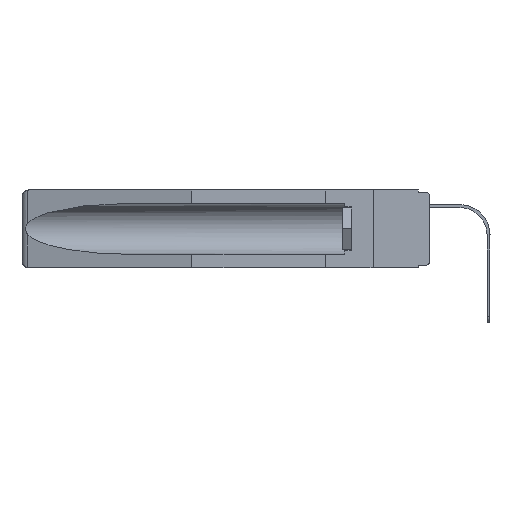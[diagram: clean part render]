
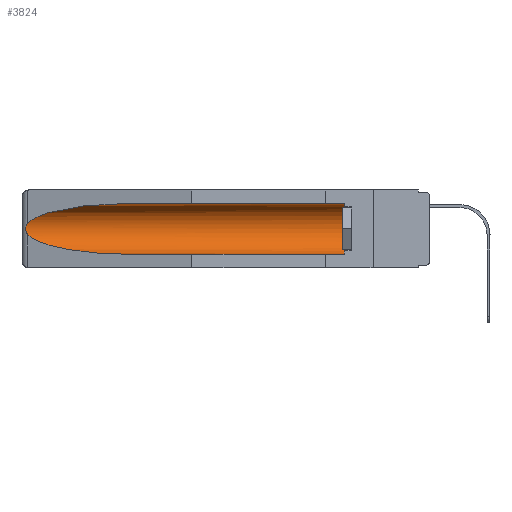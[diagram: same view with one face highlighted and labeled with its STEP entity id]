
A CAD part, left-side view. The second image highlights one B-rep face of the part: STEP entity #3824.
In plain terms, the highlighted cylindrical face has radius 2.857 mm (diameter 5.715 mm), a partial arc.
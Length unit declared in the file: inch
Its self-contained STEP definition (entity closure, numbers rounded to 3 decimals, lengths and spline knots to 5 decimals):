
#74 = LINE ( 'NONE', #165, #6207 ) ;
#165 = CARTESIAN_POINT ( 'NONE',  ( 0.155, -0.30754, -0.059 ) ) ;
#341 = CARTESIAN_POINT ( 'NONE',  ( 0.26654, 1.53092, -0.15636 ) ) ;
#357 = CARTESIAN_POINT ( 'NONE',  ( 0.26537, 1.52718, -0.19328 ) ) ;
#442 = CARTESIAN_POINT ( 'NONE',  ( 0.26597, 1.5296, -0.19026 ) ) ;
#821 = VERTEX_POINT ( 'NONE', #8668 ) ;
#824 = EDGE_CURVE ( 'NONE', #9667, #10780, #1849, .T. ) ;
#858 = ORIENTED_EDGE ( 'NONE', *, *, #10416, .T. ) ;
#1613 = CARTESIAN_POINT ( 'NONE',  ( 0.155, 0.126, -0.1715 ) ) ;
#1711 = CIRCLE ( 'NONE', #13952, 0.1125 ) ;
#1759 = CARTESIAN_POINT ( 'NONE',  ( 0.155, -0.30754, -0.284 ) ) ;
#1849 = LINE ( 'NONE', #1759, #12260 ) ;
#2006 = CARTESIAN_POINT ( 'NONE',  ( 0.26537, 1.52718, -0.19328 ) ) ;
#2422 = VERTEX_POINT ( 'NONE', #7263 ) ;
#2684 = CARTESIAN_POINT ( 'NONE',  ( 0.25451, 1.48313, -0.09465 ) ) ;
#3371 = CARTESIAN_POINT ( 'NONE',  ( 0.2673, 1.5327, -0.16383 ) ) ;
#3824 = ADVANCED_FACE ( 'NONE', ( #14123 ), #4087, .F. ) ;
#3852 = CARTESIAN_POINT ( 'NONE',  ( 0.26537, 1.52718, -0.14972 ) ) ;
#4028 = EDGE_LOOP ( 'NONE', ( #6214, #858, #6225, #10926, #14576, #13888 ) ) ;
#4059 = CARTESIAN_POINT ( 'NONE',  ( 0.21114, 1.30732, -0.059 ) ) ;
#4087 = CYLINDRICAL_SURFACE ( 'NONE', #4858, 0.1125 ) ;
#4628 = CARTESIAN_POINT ( 'NONE',  ( 0.26537, 1.52718, -0.14972 ) ) ;
#4858 = AXIS2_PLACEMENT_3D ( 'NONE', #8259, #13947, #6978 ) ;
#5714 = DIRECTION ( 'NONE',  ( 0., 1., 0. ) ) ;
#6207 = VECTOR ( 'NONE', #5714, 39.37008 ) ;
#6214 = ORIENTED_EDGE ( 'NONE', *, *, #17757, .T. ) ;
#6225 = ORIENTED_EDGE ( 'NONE', *, *, #6588, .T. ) ;
#6588 = EDGE_CURVE ( 'NONE', #14905, #10780, #17852, .T. ) ;
#6969 = DIRECTION ( 'NONE',  ( 0., -1., 0. ) ) ;
#6978 = DIRECTION ( 'NONE',  ( 0., 0., 1. ) ) ;
#7059 = CARTESIAN_POINT ( 'NONE',  ( 0.155, 1.07973, -0.284 ) ) ;
#7147 = DIRECTION ( 'NONE',  ( 0., 0., 1. ) ) ;
#7263 = CARTESIAN_POINT ( 'NONE',  ( 0.155, 0.126, -0.059 ) ) ;
#7291 = DIRECTION ( 'NONE',  ( 0., 1., 0. ) ) ;
#7539 = CARTESIAN_POINT ( 'NONE',  ( 0.26597, 1.52961, -0.15275 ) ) ;
#8259 = CARTESIAN_POINT ( 'NONE',  ( 0.155, -0.30754, -0.1715 ) ) ;
#8384 = EDGE_CURVE ( 'NONE', #2422, #821, #74, .T. ) ;
#8668 = CARTESIAN_POINT ( 'NONE',  ( 0.155, 1.07973, -0.059 ) ) ;
#8909 = CARTESIAN_POINT ( 'NONE',  ( 0.2675, 1.53308, -0.16763 ) ) ;
#9113 = B_SPLINE_CURVE_WITH_KNOTS ( 'NONE', 3,
 ( #4628, #7539, #341, #3371, #8909, #10010, #11584, #17218, #442, #2006 ),
 .UNSPECIFIED., .F., .F.,
 ( 4, 2, 2, 2, 4 ),
 ( 0., 0.00029, 0.00058, 0.00087, 0.00117 ),
 .UNSPECIFIED. ) ;
#9667 = VERTEX_POINT ( 'NONE', #11904 ) ;
#10010 = CARTESIAN_POINT ( 'NONE',  ( 0.2675, 1.53308, -0.17534 ) ) ;
#10416 = EDGE_CURVE ( 'NONE', #14748, #14905, #9113, .T. ) ;
#10512 =( BOUNDED_CURVE ( )  B_SPLINE_CURVE ( 3, ( #10984, #4059, #2684, #15266 ),
 .UNSPECIFIED., .F., .F. ) 
 B_SPLINE_CURVE_WITH_KNOTS ( ( 4, 4 ),
 ( 4.71239, 6.08839 ),
 .UNSPECIFIED. ) 
 CURVE ( )  GEOMETRIC_REPRESENTATION_ITEM ( )  RATIONAL_B_SPLINE_CURVE ( ( 1., 0.848, 0.848, 1. ) ) 
 REPRESENTATION_ITEM ( '' )  );
#10780 = VERTEX_POINT ( 'NONE', #7059 ) ;
#10926 = ORIENTED_EDGE ( 'NONE', *, *, #824, .F. ) ;
#10984 = CARTESIAN_POINT ( 'NONE',  ( 0.155, 1.07973, -0.059 ) ) ;
#11584 = CARTESIAN_POINT ( 'NONE',  ( 0.2673, 1.53269, -0.17917 ) ) ;
#11904 = CARTESIAN_POINT ( 'NONE',  ( 0.155, 0.126, -0.284 ) ) ;
#12260 = VECTOR ( 'NONE', #7291, 39.37008 ) ;
#12422 = CARTESIAN_POINT ( 'NONE',  ( 0.26537, 1.52718, -0.19328 ) ) ;
#13116 = EDGE_CURVE ( 'NONE', #9667, #2422, #1711, .T. ) ;
#13888 = ORIENTED_EDGE ( 'NONE', *, *, #8384, .T. ) ;
#13947 = DIRECTION ( 'NONE',  ( 0., 1., 0. ) ) ;
#13952 = AXIS2_PLACEMENT_3D ( 'NONE', #1613, #6969, #7147 ) ;
#14123 = FACE_OUTER_BOUND ( 'NONE', #4028, .T. ) ;
#14576 = ORIENTED_EDGE ( 'NONE', *, *, #13116, .T. ) ;
#14748 = VERTEX_POINT ( 'NONE', #3852 ) ;
#14819 = CARTESIAN_POINT ( 'NONE',  ( 0.155, 1.07973, -0.284 ) ) ;
#14905 = VERTEX_POINT ( 'NONE', #357 ) ;
#15266 = CARTESIAN_POINT ( 'NONE',  ( 0.26537, 1.52718, -0.14972 ) ) ;
#16611 = CARTESIAN_POINT ( 'NONE',  ( 0.21114, 1.30732, -0.284 ) ) ;
#17218 = CARTESIAN_POINT ( 'NONE',  ( 0.26655, 1.53094, -0.18657 ) ) ;
#17757 = EDGE_CURVE ( 'NONE', #821, #14748, #10512, .T. ) ;
#17852 =( BOUNDED_CURVE ( )  B_SPLINE_CURVE ( 3, ( #12422, #17970, #16611, #14819 ),
 .UNSPECIFIED., .F., .F. ) 
 B_SPLINE_CURVE_WITH_KNOTS ( ( 4, 4 ),
 ( 0.1948, 1.5708 ),
 .UNSPECIFIED. ) 
 CURVE ( )  GEOMETRIC_REPRESENTATION_ITEM ( )  RATIONAL_B_SPLINE_CURVE ( ( 1., 0.848, 0.848, 1. ) ) 
 REPRESENTATION_ITEM ( '' )  );
#17970 = CARTESIAN_POINT ( 'NONE',  ( 0.25451, 1.48313, -0.24835 ) ) ;
